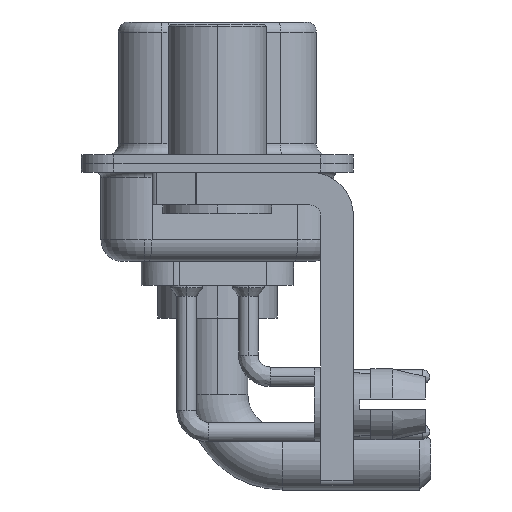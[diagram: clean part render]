
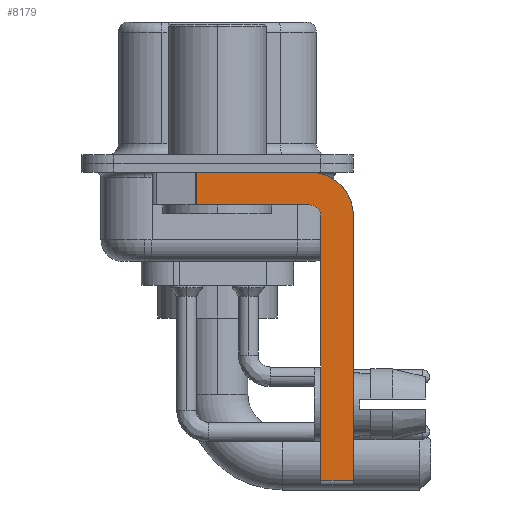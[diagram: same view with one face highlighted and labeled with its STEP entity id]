
A CAD part, left-side view. The second image highlights one B-rep face of the part: STEP entity #8179.
In plain terms, the highlighted planar face has unit normal (-1, 0, 0).
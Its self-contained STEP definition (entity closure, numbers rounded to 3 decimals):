
#133 = CARTESIAN_POINT ( 'NONE',  ( -2.9, 3., -0.4 ) ) ;
#696 = EDGE_CURVE ( 'NONE', #6005, #1278, #24541, .T. ) ;
#951 = ORIENTED_EDGE ( 'NONE', *, *, #1289, .F. ) ;
#1278 = VERTEX_POINT ( 'NONE', #5227 ) ;
#1289 = EDGE_CURVE ( 'NONE', #10314, #6005, #4066, .T. ) ;
#2314 = VECTOR ( 'NONE', #9678, 1000. ) ;
#2514 = CARTESIAN_POINT ( 'NONE',  ( -2.9, -4.25, -0.4 ) ) ;
#2900 = CARTESIAN_POINT ( 'NONE',  ( -2.9, -6.25, -2.4 ) ) ;
#4066 = CIRCLE ( 'NONE', #20360, 0.5 ) ;
#4199 = LINE ( 'NONE', #133, #5965 ) ;
#4355 = DIRECTION ( 'NONE',  ( 1., 0., 0. ) ) ;
#4493 = CARTESIAN_POINT ( 'NONE',  ( -2.9, 0.978, -0.4 ) ) ;
#4661 = VERTEX_POINT ( 'NONE', #2900 ) ;
#4857 = CARTESIAN_POINT ( 'NONE',  ( -2.9, -4.25, -14.55 ) ) ;
#5227 = CARTESIAN_POINT ( 'NONE',  ( -2.9, 0.978, -1.9 ) ) ;
#5331 = ORIENTED_EDGE ( 'NONE', *, *, #10642, .F. ) ;
#5577 = VERTEX_POINT ( 'NONE', #4493 ) ;
#5965 = VECTOR ( 'NONE', #18342, 1000. ) ;
#6005 = VERTEX_POINT ( 'NONE', #23513 ) ;
#6377 = DIRECTION ( 'NONE',  ( 0., 0., -1. ) ) ;
#6624 = CARTESIAN_POINT ( 'NONE',  ( -2.9, 0.978, -1.9 ) ) ;
#6690 = CARTESIAN_POINT ( 'NONE',  ( -2.9, -4.25, -1.9 ) ) ;
#7210 = LINE ( 'NONE', #4857, #2314 ) ;
#7287 = EDGE_CURVE ( 'NONE', #5577, #1278, #24597, .T. ) ;
#7308 = VECTOR ( 'NONE', #22624, 1000. ) ;
#7398 = EDGE_CURVE ( 'NONE', #15882, #10314, #13186, .T. ) ;
#7722 = CARTESIAN_POINT ( 'NONE',  ( -2.9, -6.25, -14.55 ) ) ;
#7796 = ORIENTED_EDGE ( 'NONE', *, *, #16575, .T. ) ;
#8179 = ADVANCED_FACE ( 'NONE', ( #16663 ), #22832, .F. ) ;
#8819 = ORIENTED_EDGE ( 'NONE', *, *, #9896, .F. ) ;
#8888 = CARTESIAN_POINT ( 'NONE',  ( -2.9, -4.25, -2.4 ) ) ;
#9484 = ORIENTED_EDGE ( 'NONE', *, *, #7287, .T. ) ;
#9678 = DIRECTION ( 'NONE',  ( 0., -1., 0. ) ) ;
#9814 = DIRECTION ( 'NONE',  ( -1., 0., 0. ) ) ;
#9896 = EDGE_CURVE ( 'NONE', #4661, #13328, #14659, .T. ) ;
#9954 = CARTESIAN_POINT ( 'NONE',  ( -2.9, -4.25, -2.4 ) ) ;
#10314 = VERTEX_POINT ( 'NONE', #15277 ) ;
#10642 = EDGE_CURVE ( 'NONE', #5577, #12151, #4199, .T. ) ;
#10920 = VECTOR ( 'NONE', #22799, 1000. ) ;
#11365 = AXIS2_PLACEMENT_3D ( 'NONE', #20588, #4355, #12342 ) ;
#12151 = VERTEX_POINT ( 'NONE', #2514 ) ;
#12342 = DIRECTION ( 'NONE',  ( 0., 0., -1. ) ) ;
#13186 = LINE ( 'NONE', #21587, #25757 ) ;
#13328 = VERTEX_POINT ( 'NONE', #7722 ) ;
#13716 = CARTESIAN_POINT ( 'NONE',  ( -2.9, -4.75, -14.55 ) ) ;
#13878 = DIRECTION ( 'NONE',  ( 0., 0., 1. ) ) ;
#14636 = EDGE_LOOP ( 'NONE', ( #5331, #9484, #16362, #951, #23382, #7796, #8819, #25349 ) ) ;
#14659 = LINE ( 'NONE', #24269, #10920 ) ;
#14686 = DIRECTION ( 'NONE',  ( 0., 1., 0. ) ) ;
#15277 = CARTESIAN_POINT ( 'NONE',  ( -2.9, -4.75, -2.4 ) ) ;
#15543 = DIRECTION ( 'NONE',  ( 0., 0., 1. ) ) ;
#15882 = VERTEX_POINT ( 'NONE', #13716 ) ;
#16362 = ORIENTED_EDGE ( 'NONE', *, *, #696, .F. ) ;
#16575 = EDGE_CURVE ( 'NONE', #15882, #13328, #7210, .T. ) ;
#16663 = FACE_OUTER_BOUND ( 'NONE', #14636, .T. ) ;
#17814 = VECTOR ( 'NONE', #14686, 1000. ) ;
#18342 = DIRECTION ( 'NONE',  ( 0., -1., 0. ) ) ;
#20061 = EDGE_CURVE ( 'NONE', #12151, #4661, #25195, .T. ) ;
#20164 = AXIS2_PLACEMENT_3D ( 'NONE', #9954, #24239, #6377 ) ;
#20360 = AXIS2_PLACEMENT_3D ( 'NONE', #8888, #9814, #13878 ) ;
#20588 = CARTESIAN_POINT ( 'NONE',  ( -2.9, -4.25, -2.4 ) ) ;
#21587 = CARTESIAN_POINT ( 'NONE',  ( -2.9, -4.75, -14.8 ) ) ;
#22624 = DIRECTION ( 'NONE',  ( 0., 0., -1. ) ) ;
#22799 = DIRECTION ( 'NONE',  ( 0., 0., -1. ) ) ;
#22832 = PLANE ( 'NONE',  #11365 ) ;
#23382 = ORIENTED_EDGE ( 'NONE', *, *, #7398, .F. ) ;
#23513 = CARTESIAN_POINT ( 'NONE',  ( -2.9, -4.25, -1.9 ) ) ;
#24239 = DIRECTION ( 'NONE',  ( 1., 0., 0. ) ) ;
#24269 = CARTESIAN_POINT ( 'NONE',  ( -2.9, -6.25, -2.4 ) ) ;
#24541 = LINE ( 'NONE', #6690, #17814 ) ;
#24597 = LINE ( 'NONE', #6624, #7308 ) ;
#25195 = CIRCLE ( 'NONE', #20164, 2. ) ;
#25349 = ORIENTED_EDGE ( 'NONE', *, *, #20061, .F. ) ;
#25757 = VECTOR ( 'NONE', #15543, 1000. ) ;
